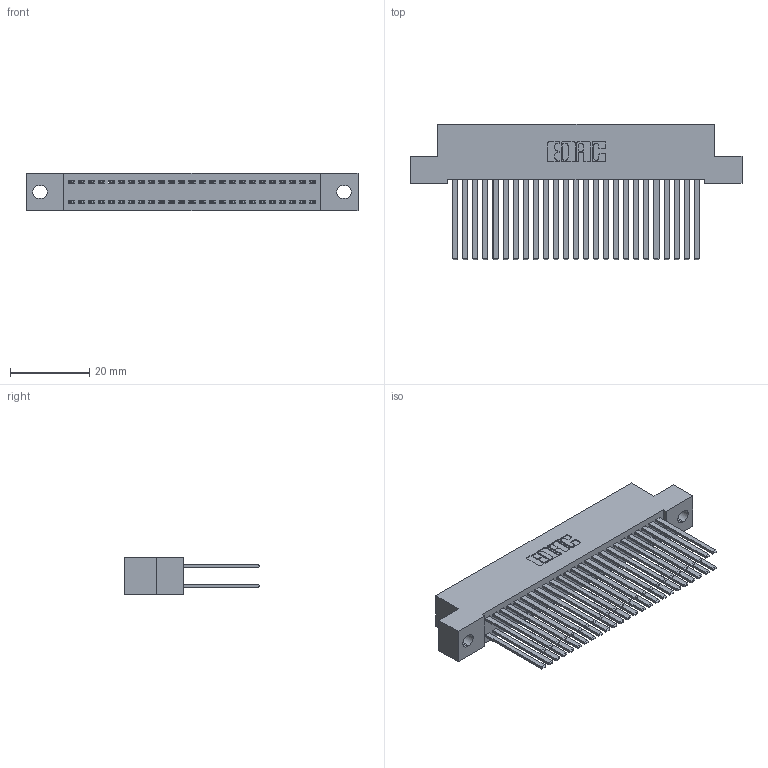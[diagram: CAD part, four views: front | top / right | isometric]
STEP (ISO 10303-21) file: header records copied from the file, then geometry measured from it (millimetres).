
FILE_DESCRIPTION (( 'STEP AP203' ), '1' );
FILE_NAME ('342-050-544-202.STEP', '2019-10-02T23:53:31', ( '' ), ( '' ), 'SwSTEP 2.0', 'SolidWorks 2016', '' );
FILE_SCHEMA (( 'CONFIG_CONTROL_DESIGN' ));
Length unit declared in the file: inch
Products named in the file (3): 342 Part_.128 Slot; 345-292-001_345-293-144; 342-050-544-202
Assembly tree (51 placements, depth 2):
  342-050-544-202
    342 Part_.128 Slot
    345-292-001_345-293-144  x50
Bounding box: 83.82 x 34.3 x 9.4 mm (x, y, z)
Volume: 8099.5 mm3; surface area: 14465.6 mm2
Topology: 51 solids, 51 shells, 2414 faces, 7161 edges, 4706 vertices
Faces by surface type: plane 1670, cylinder 744
Entity records: 18101 total; most frequent: CARTESIAN_POINT 3018, ORIENTED_EDGE 2954, DIRECTION 2605, EDGE_CURVE 1477, LINE 1353, VECTOR 1353, VERTEX_POINT 982, AXIS2_PLACEMENT_3D 626
